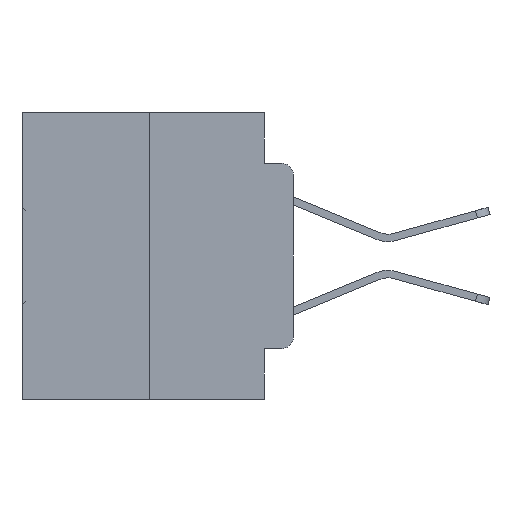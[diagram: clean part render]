
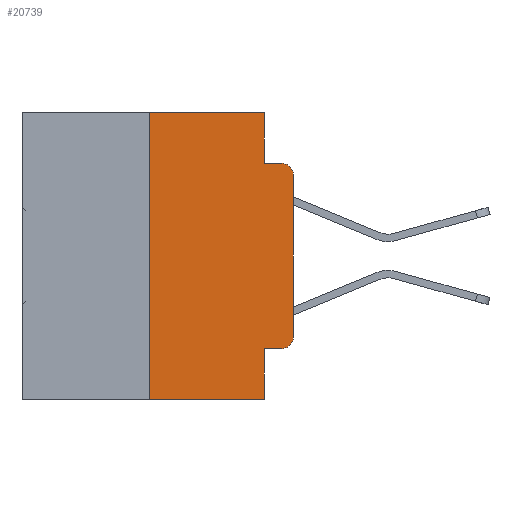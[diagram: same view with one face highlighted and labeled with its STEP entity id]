
A CAD part, left-side view. The second image highlights one B-rep face of the part: STEP entity #20739.
In plain terms, the highlighted planar face has unit normal (-1, 0, 0).
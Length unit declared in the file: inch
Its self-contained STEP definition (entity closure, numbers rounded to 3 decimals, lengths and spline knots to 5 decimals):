
#34 = CARTESIAN_POINT ( 'NONE',  ( 0., 0.051, -0.5 ) ) ;
#264 = DIRECTION ( 'NONE',  ( 0., 0., 1. ) ) ;
#333 = EDGE_CURVE ( 'NONE', #5379, #25732, #17534, .T. ) ;
#334 = VERTEX_POINT ( 'NONE', #30359 ) ;
#584 = DIRECTION ( 'NONE',  ( 1., 0., 0. ) ) ;
#901 = VERTEX_POINT ( 'NONE', #15016 ) ;
#1351 = CARTESIAN_POINT ( 'NONE',  ( 0., 0.25, -0.5 ) ) ;
#1993 = VECTOR ( 'NONE', #29149, 39.37008 ) ;
#2174 = LINE ( 'NONE', #31242, #19166 ) ;
#2304 = EDGE_CURVE ( 'NONE', #11704, #30231, #21733, .T. ) ;
#2605 = EDGE_LOOP ( 'NONE', ( #3188, #19339, #27661, #15405, #17011, #13384, #21740, #31613, #8547, #13412 ) ) ;
#2939 = VECTOR ( 'NONE', #13643, 39.37008 ) ;
#3188 = ORIENTED_EDGE ( 'NONE', *, *, #17178, .T. ) ;
#3221 = DIRECTION ( 'NONE',  ( 0., -1., 0. ) ) ;
#3803 = CARTESIAN_POINT ( 'NONE',  ( 0., 0.02, -0.4115 ) ) ;
#4050 = LINE ( 'NONE', #15883, #29668 ) ;
#4626 = VECTOR ( 'NONE', #25698, 39.37008 ) ;
#5379 = VERTEX_POINT ( 'NONE', #16975 ) ;
#6172 = VERTEX_POINT ( 'NONE', #22675 ) ;
#7335 = EDGE_CURVE ( 'NONE', #334, #31129, #16124, .T. ) ;
#8547 = ORIENTED_EDGE ( 'NONE', *, *, #7335, .T. ) ;
#9246 = VECTOR ( 'NONE', #12601, 39.37008 ) ;
#9672 = CARTESIAN_POINT ( 'NONE',  ( 0., 0.02, -0.1085 ) ) ;
#10421 = CARTESIAN_POINT ( 'NONE',  ( 0., 0.473, 0. ) ) ;
#10580 = VECTOR ( 'NONE', #3221, 39.37008 ) ;
#10926 = DIRECTION ( 'NONE',  ( 0., 0., -1. ) ) ;
#11133 = VERTEX_POINT ( 'NONE', #32495 ) ;
#11315 = CIRCLE ( 'NONE', #26536, 0.02 ) ;
#11491 = EDGE_CURVE ( 'NONE', #25732, #901, #17446, .T. ) ;
#11704 = VERTEX_POINT ( 'NONE', #1351 ) ;
#11777 = DIRECTION ( 'NONE',  ( -1., 0., 0. ) ) ;
#12291 = DIRECTION ( 'NONE',  ( 0., 0., -1. ) ) ;
#12491 = VECTOR ( 'NONE', #21839, 39.37008 ) ;
#12601 = DIRECTION ( 'NONE',  ( 0., -1., 0. ) ) ;
#12773 = EDGE_CURVE ( 'NONE', #11704, #11133, #14101, .T. ) ;
#13384 = ORIENTED_EDGE ( 'NONE', *, *, #12773, .F. ) ;
#13412 = ORIENTED_EDGE ( 'NONE', *, *, #18424, .T. ) ;
#13643 = DIRECTION ( 'NONE',  ( 0., 0., -1. ) ) ;
#13684 = CARTESIAN_POINT ( 'NONE',  ( 0., 0.051, 0. ) ) ;
#14101 = LINE ( 'NONE', #16779, #12491 ) ;
#14172 = CARTESIAN_POINT ( 'NONE',  ( 0., 0., -0.1085 ) ) ;
#14767 = EDGE_CURVE ( 'NONE', #334, #30231, #2174, .T. ) ;
#15016 = CARTESIAN_POINT ( 'NONE',  ( 0., 0.02, -0.0885 ) ) ;
#15073 = EDGE_CURVE ( 'NONE', #27232, #901, #27455, .T. ) ;
#15405 = ORIENTED_EDGE ( 'NONE', *, *, #333, .F. ) ;
#15883 = CARTESIAN_POINT ( 'NONE',  ( 0., 0., 0. ) ) ;
#16124 = LINE ( 'NONE', #27819, #9246 ) ;
#16193 = CARTESIAN_POINT ( 'NONE',  ( 0., 0.473, 0. ) ) ;
#16779 = CARTESIAN_POINT ( 'NONE',  ( 0., 0.25, 0. ) ) ;
#16975 = CARTESIAN_POINT ( 'NONE',  ( 0., 0.051, 0. ) ) ;
#17011 = ORIENTED_EDGE ( 'NONE', *, *, #32141, .F. ) ;
#17178 = EDGE_CURVE ( 'NONE', #6172, #27232, #4050, .T. ) ;
#17446 = LINE ( 'NONE', #21122, #10580 ) ;
#17534 = LINE ( 'NONE', #13684, #2939 ) ;
#18111 = AXIS2_PLACEMENT_3D ( 'NONE', #16193, #584, #18746 ) ;
#18424 = EDGE_CURVE ( 'NONE', #31129, #6172, #11315, .T. ) ;
#18746 = DIRECTION ( 'NONE',  ( 0., 0., -1. ) ) ;
#19138 = LINE ( 'NONE', #10421, #4626 ) ;
#19166 = VECTOR ( 'NONE', #10926, 39.37008 ) ;
#19339 = ORIENTED_EDGE ( 'NONE', *, *, #15073, .T. ) ;
#19887 = AXIS2_PLACEMENT_3D ( 'NONE', #9672, #27510, #12291 ) ;
#20739 = ADVANCED_FACE ( 'NONE', ( #25524 ), #28791, .F. ) ;
#21122 = CARTESIAN_POINT ( 'NONE',  ( 0., 0.051, -0.0885 ) ) ;
#21733 = LINE ( 'NONE', #29390, #1993 ) ;
#21740 = ORIENTED_EDGE ( 'NONE', *, *, #2304, .T. ) ;
#21839 = DIRECTION ( 'NONE',  ( 0., 0., 1. ) ) ;
#22675 = CARTESIAN_POINT ( 'NONE',  ( 0., 0., -0.3915 ) ) ;
#24161 = CARTESIAN_POINT ( 'NONE',  ( 0., 0.051, -0.0885 ) ) ;
#25524 = FACE_OUTER_BOUND ( 'NONE', #2605, .T. ) ;
#25698 = DIRECTION ( 'NONE',  ( 0., -1., 0. ) ) ;
#25732 = VERTEX_POINT ( 'NONE', #24161 ) ;
#26536 = AXIS2_PLACEMENT_3D ( 'NONE', #27022, #11777, #29545 ) ;
#27022 = CARTESIAN_POINT ( 'NONE',  ( 0., 0.02, -0.3915 ) ) ;
#27232 = VERTEX_POINT ( 'NONE', #14172 ) ;
#27455 = CIRCLE ( 'NONE', #19887, 0.02 ) ;
#27510 = DIRECTION ( 'NONE',  ( -1., 0., 0. ) ) ;
#27661 = ORIENTED_EDGE ( 'NONE', *, *, #11491, .F. ) ;
#27819 = CARTESIAN_POINT ( 'NONE',  ( 0., 0.051, -0.4115 ) ) ;
#28791 = PLANE ( 'NONE',  #18111 ) ;
#29149 = DIRECTION ( 'NONE',  ( 0., -1., 0. ) ) ;
#29390 = CARTESIAN_POINT ( 'NONE',  ( 0., 0.473, -0.5 ) ) ;
#29545 = DIRECTION ( 'NONE',  ( 0., 0., -1. ) ) ;
#29668 = VECTOR ( 'NONE', #264, 39.37008 ) ;
#30231 = VERTEX_POINT ( 'NONE', #34 ) ;
#30359 = CARTESIAN_POINT ( 'NONE',  ( 0., 0.051, -0.4115 ) ) ;
#31129 = VERTEX_POINT ( 'NONE', #3803 ) ;
#31242 = CARTESIAN_POINT ( 'NONE',  ( 0., 0.051, 0. ) ) ;
#31613 = ORIENTED_EDGE ( 'NONE', *, *, #14767, .F. ) ;
#32141 = EDGE_CURVE ( 'NONE', #11133, #5379, #19138, .T. ) ;
#32495 = CARTESIAN_POINT ( 'NONE',  ( 0., 0.25, 0. ) ) ;
